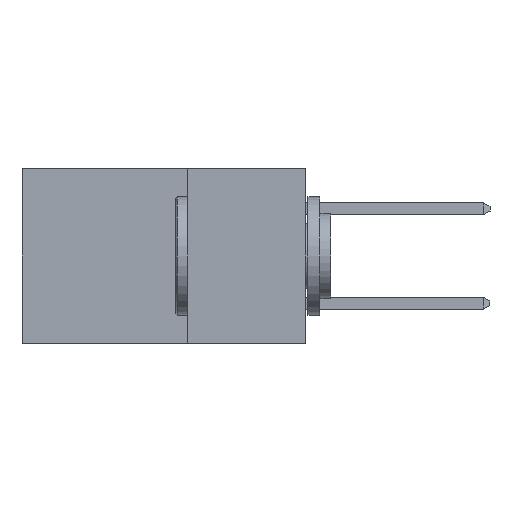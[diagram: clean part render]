
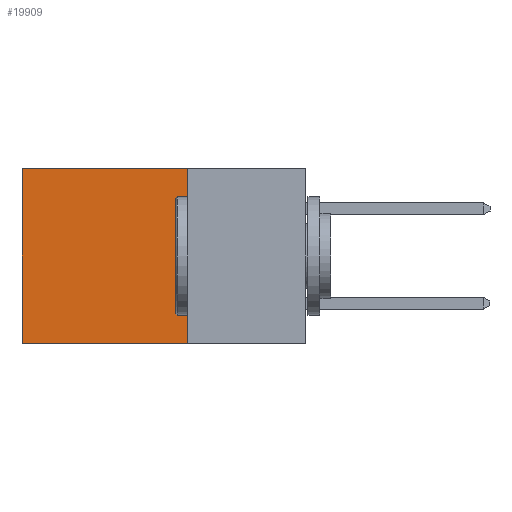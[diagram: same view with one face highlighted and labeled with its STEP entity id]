
A CAD part, left-side view. The second image highlights one B-rep face of the part: STEP entity #19909.
In plain terms, the highlighted planar face has unit normal (-1, 0, 0).
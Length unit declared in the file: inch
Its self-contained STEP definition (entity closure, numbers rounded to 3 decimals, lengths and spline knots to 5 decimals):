
#1581 = DIRECTION ( 'NONE',  ( 0., 0., -1. ) ) ;
#2578 = DIRECTION ( 'NONE',  ( 0., 0., -1. ) ) ;
#3141 = EDGE_CURVE ( 'NONE', #17842, #7635, #4622, .T. ) ;
#3791 = ORIENTED_EDGE ( 'NONE', *, *, #3141, .T. ) ;
#4622 = LINE ( 'NONE', #6879, #14453 ) ;
#4661 = EDGE_CURVE ( 'NONE', #17842, #10363, #5462, .T. ) ;
#4920 = VERTEX_POINT ( 'NONE', #12173 ) ;
#4980 = EDGE_CURVE ( 'NONE', #7635, #4920, #13744, .T. ) ;
#5449 = FACE_OUTER_BOUND ( 'NONE', #18743, .T. ) ;
#5462 = LINE ( 'NONE', #14729, #10768 ) ;
#6193 = AXIS2_PLACEMENT_3D ( 'NONE', #24593, #13330, #1581 ) ;
#6879 = CARTESIAN_POINT ( 'NONE',  ( 0.298, 0.25, 0. ) ) ;
#7635 = VERTEX_POINT ( 'NONE', #10263 ) ;
#8717 = DIRECTION ( 'NONE',  ( 0., 1., 0. ) ) ;
#8748 = CARTESIAN_POINT ( 'NONE',  ( 0.298, 0.25, -0.37 ) ) ;
#8753 = CARTESIAN_POINT ( 'NONE',  ( 0.298, 0.25, 0. ) ) ;
#9122 = LINE ( 'NONE', #8748, #18747 ) ;
#10263 = CARTESIAN_POINT ( 'NONE',  ( 0.298, 0.6, 0. ) ) ;
#10363 = VERTEX_POINT ( 'NONE', #17757 ) ;
#10767 = DIRECTION ( 'NONE',  ( 0., 1., 0. ) ) ;
#10768 = VECTOR ( 'NONE', #2578, 39.37008 ) ;
#11071 = DIRECTION ( 'NONE',  ( 0., 0., -1. ) ) ;
#11419 = PLANE ( 'NONE',  #6193 ) ;
#12173 = CARTESIAN_POINT ( 'NONE',  ( 0.298, 0.6, -0.37 ) ) ;
#13321 = CARTESIAN_POINT ( 'NONE',  ( 0.298, 0.6, 0. ) ) ;
#13330 = DIRECTION ( 'NONE',  ( 1., 0., 0. ) ) ;
#13744 = LINE ( 'NONE', #13321, #22653 ) ;
#14453 = VECTOR ( 'NONE', #8717, 39.37008 ) ;
#14729 = CARTESIAN_POINT ( 'NONE',  ( 0.298, 0.25, 0. ) ) ;
#16464 = ORIENTED_EDGE ( 'NONE', *, *, #4661, .F. ) ;
#17757 = CARTESIAN_POINT ( 'NONE',  ( 0.298, 0.25, -0.37 ) ) ;
#17842 = VERTEX_POINT ( 'NONE', #8753 ) ;
#18053 = ORIENTED_EDGE ( 'NONE', *, *, #21072, .F. ) ;
#18743 = EDGE_LOOP ( 'NONE', ( #20848, #18053, #16464, #3791 ) ) ;
#18747 = VECTOR ( 'NONE', #10767, 39.37008 ) ;
#19909 = ADVANCED_FACE ( 'NONE', ( #5449 ), #11419, .F. ) ;
#20848 = ORIENTED_EDGE ( 'NONE', *, *, #4980, .T. ) ;
#21072 = EDGE_CURVE ( 'NONE', #10363, #4920, #9122, .T. ) ;
#22653 = VECTOR ( 'NONE', #11071, 39.37008 ) ;
#24593 = CARTESIAN_POINT ( 'NONE',  ( 0.298, 0.25, 0. ) ) ;
